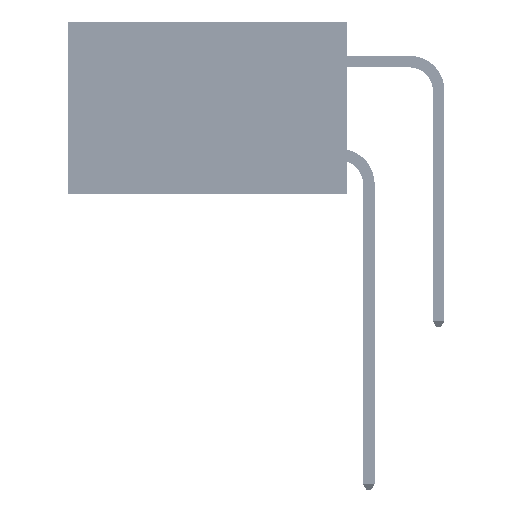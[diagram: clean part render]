
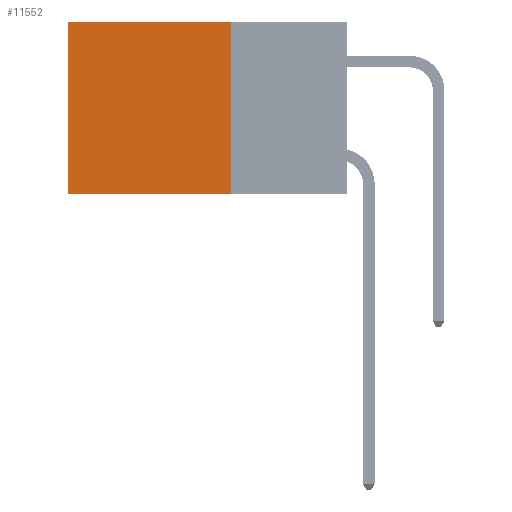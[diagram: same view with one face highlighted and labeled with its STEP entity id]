
A CAD part, left-side view. The second image highlights one B-rep face of the part: STEP entity #11552.
In plain terms, the highlighted planar face has unit normal (-1, 0, 0).
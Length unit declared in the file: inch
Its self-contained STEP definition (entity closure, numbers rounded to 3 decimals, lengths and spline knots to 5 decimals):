
#1935 = VERTEX_POINT ( 'NONE', #20036 ) ;
#5501 = DIRECTION ( 'NONE',  ( 0., 0., -1. ) ) ;
#6285 = VECTOR ( 'NONE', #16975, 39.37008 ) ;
#8057 = ORIENTED_EDGE ( 'NONE', *, *, #36709, .F. ) ;
#8199 = EDGE_CURVE ( 'NONE', #11628, #21874, #16396, .T. ) ;
#8360 = AXIS2_PLACEMENT_3D ( 'NONE', #11427, #37754, #15257 ) ;
#10801 = ORIENTED_EDGE ( 'NONE', *, *, #8199, .T. ) ;
#11199 = CARTESIAN_POINT ( 'NONE',  ( 0.2875, 0.6, -0.37 ) ) ;
#11427 = CARTESIAN_POINT ( 'NONE',  ( 0.2875, 0.25, 0. ) ) ;
#11552 = ADVANCED_FACE ( 'NONE', ( #36996 ), #34030, .F. ) ;
#11628 = VERTEX_POINT ( 'NONE', #11756 ) ;
#11756 = CARTESIAN_POINT ( 'NONE',  ( 0.2875, 0.25, 0. ) ) ;
#15257 = DIRECTION ( 'NONE',  ( 0., 0., -1. ) ) ;
#16396 = LINE ( 'NONE', #35709, #6285 ) ;
#16975 = DIRECTION ( 'NONE',  ( 0., 1., 0. ) ) ;
#17976 = VECTOR ( 'NONE', #28721, 39.37008 ) ;
#17986 = CARTESIAN_POINT ( 'NONE',  ( 0.2875, 0.25, 0. ) ) ;
#18731 = EDGE_LOOP ( 'NONE', ( #25685, #8057, #45579, #10801 ) ) ;
#19717 = VECTOR ( 'NONE', #44230, 39.37008 ) ;
#20036 = CARTESIAN_POINT ( 'NONE',  ( 0.2875, 0.25, -0.37 ) ) ;
#21874 = VERTEX_POINT ( 'NONE', #27651 ) ;
#25685 = ORIENTED_EDGE ( 'NONE', *, *, #39825, .T. ) ;
#27651 = CARTESIAN_POINT ( 'NONE',  ( 0.2875, 0.6, 0. ) ) ;
#28003 = LINE ( 'NONE', #39677, #17976 ) ;
#28175 = CARTESIAN_POINT ( 'NONE',  ( 0.2875, 0.6, 0. ) ) ;
#28721 = DIRECTION ( 'NONE',  ( 0., 1., 0. ) ) ;
#34030 = PLANE ( 'NONE',  #8360 ) ;
#35709 = CARTESIAN_POINT ( 'NONE',  ( 0.2875, 0.25, 0. ) ) ;
#36709 = EDGE_CURVE ( 'NONE', #1935, #41745, #28003, .T. ) ;
#36996 = FACE_OUTER_BOUND ( 'NONE', #18731, .T. ) ;
#37754 = DIRECTION ( 'NONE',  ( 1., 0., 0. ) ) ;
#39677 = CARTESIAN_POINT ( 'NONE',  ( 0.2875, 0.25, -0.37 ) ) ;
#39825 = EDGE_CURVE ( 'NONE', #21874, #41745, #40662, .T. ) ;
#40662 = LINE ( 'NONE', #28175, #47064 ) ;
#41745 = VERTEX_POINT ( 'NONE', #11199 ) ;
#44230 = DIRECTION ( 'NONE',  ( 0., 0., -1. ) ) ;
#45164 = EDGE_CURVE ( 'NONE', #11628, #1935, #48447, .T. ) ;
#45579 = ORIENTED_EDGE ( 'NONE', *, *, #45164, .F. ) ;
#47064 = VECTOR ( 'NONE', #5501, 39.37008 ) ;
#48447 = LINE ( 'NONE', #17986, #19717 ) ;
